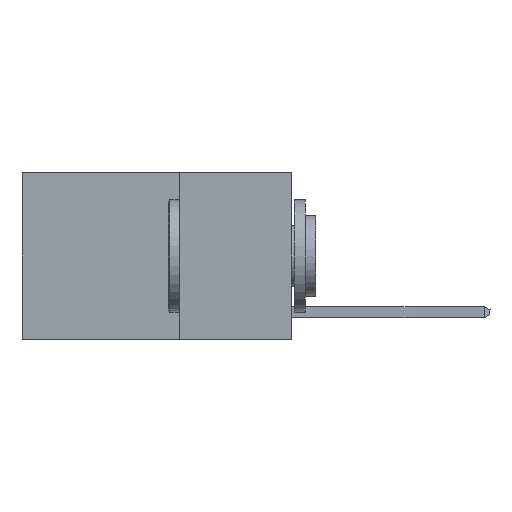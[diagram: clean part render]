
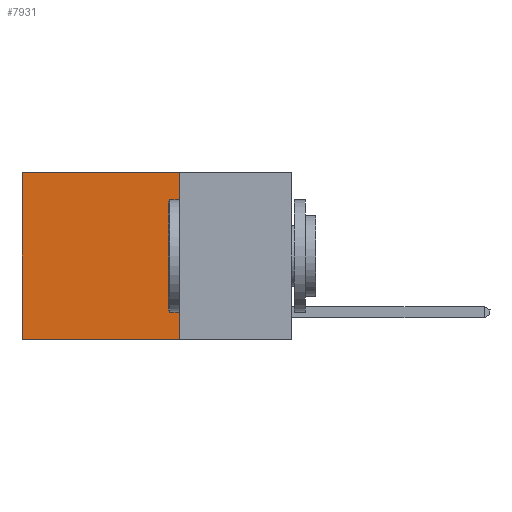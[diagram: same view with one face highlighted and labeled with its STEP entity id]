
A CAD part, left-side view. The second image highlights one B-rep face of the part: STEP entity #7931.
In plain terms, the highlighted planar face has unit normal (-1, 0, 0).
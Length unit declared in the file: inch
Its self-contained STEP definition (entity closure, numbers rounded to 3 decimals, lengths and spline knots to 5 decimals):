
#328 = CARTESIAN_POINT ( 'NONE',  ( 0.2625, 0.6, 0. ) ) ;
#1224 = ORIENTED_EDGE ( 'NONE', *, *, #4033, .F. ) ;
#1336 = LINE ( 'NONE', #13746, #18748 ) ;
#2052 = EDGE_CURVE ( 'NONE', #4573, #17069, #2535, .T. ) ;
#2535 = LINE ( 'NONE', #11861, #17147 ) ;
#4033 = EDGE_CURVE ( 'NONE', #14109, #12329, #13926, .T. ) ;
#4402 = VECTOR ( 'NONE', #15337, 39.37008 ) ;
#4573 = VERTEX_POINT ( 'NONE', #328 ) ;
#4804 = DIRECTION ( 'NONE',  ( 0., 0., -1. ) ) ;
#4942 = ORIENTED_EDGE ( 'NONE', *, *, #12192, .F. ) ;
#5771 = CARTESIAN_POINT ( 'NONE',  ( 0.2625, 0.25, 0. ) ) ;
#6427 = DIRECTION ( 'NONE',  ( 0., 1., 0. ) ) ;
#7615 = DIRECTION ( 'NONE',  ( 0., 0., -1. ) ) ;
#7931 = ADVANCED_FACE ( 'NONE', ( #14938 ), #13844, .F. ) ;
#8279 = VECTOR ( 'NONE', #8648, 39.37008 ) ;
#8596 = LINE ( 'NONE', #10899, #4402 ) ;
#8648 = DIRECTION ( 'NONE',  ( 0., 0., -1. ) ) ;
#9495 = CARTESIAN_POINT ( 'NONE',  ( 0.2625, 0.6, -0.37 ) ) ;
#10899 = CARTESIAN_POINT ( 'NONE',  ( 0.2625, 0.25, 0. ) ) ;
#11242 = CARTESIAN_POINT ( 'NONE',  ( 0.2625, 0.25, -0.37 ) ) ;
#11277 = AXIS2_PLACEMENT_3D ( 'NONE', #18489, #12538, #4804 ) ;
#11861 = CARTESIAN_POINT ( 'NONE',  ( 0.2625, 0.6, 0. ) ) ;
#11865 = ORIENTED_EDGE ( 'NONE', *, *, #2052, .T. ) ;
#12171 = EDGE_LOOP ( 'NONE', ( #11865, #4942, #1224, #17462 ) ) ;
#12192 = EDGE_CURVE ( 'NONE', #12329, #17069, #1336, .T. ) ;
#12329 = VERTEX_POINT ( 'NONE', #11242 ) ;
#12538 = DIRECTION ( 'NONE',  ( 1., 0., 0. ) ) ;
#13746 = CARTESIAN_POINT ( 'NONE',  ( 0.2625, 0.25, -0.37 ) ) ;
#13844 = PLANE ( 'NONE',  #11277 ) ;
#13926 = LINE ( 'NONE', #5771, #8279 ) ;
#14109 = VERTEX_POINT ( 'NONE', #17867 ) ;
#14406 = EDGE_CURVE ( 'NONE', #14109, #4573, #8596, .T. ) ;
#14938 = FACE_OUTER_BOUND ( 'NONE', #12171, .T. ) ;
#15337 = DIRECTION ( 'NONE',  ( 0., 1., 0. ) ) ;
#17069 = VERTEX_POINT ( 'NONE', #9495 ) ;
#17147 = VECTOR ( 'NONE', #7615, 39.37008 ) ;
#17462 = ORIENTED_EDGE ( 'NONE', *, *, #14406, .T. ) ;
#17867 = CARTESIAN_POINT ( 'NONE',  ( 0.2625, 0.25, 0. ) ) ;
#18489 = CARTESIAN_POINT ( 'NONE',  ( 0.2625, 0.25, 0. ) ) ;
#18748 = VECTOR ( 'NONE', #6427, 39.37008 ) ;
